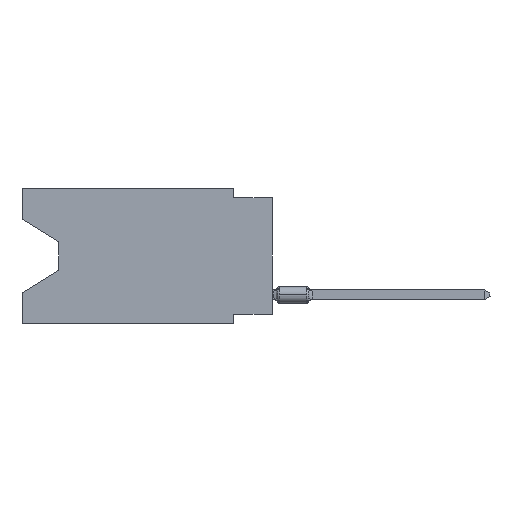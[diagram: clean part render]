
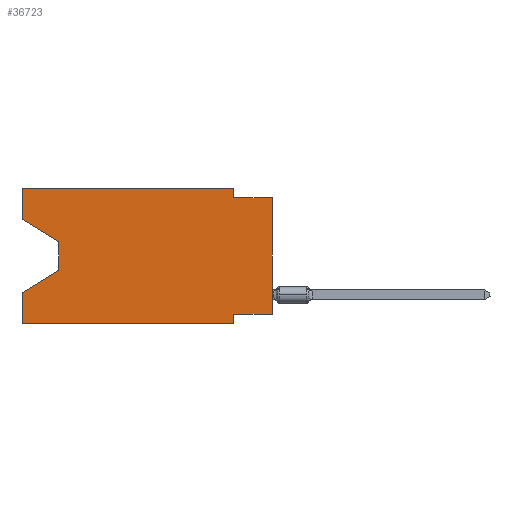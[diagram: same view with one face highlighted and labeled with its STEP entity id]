
A CAD part, left-side view. The second image highlights one B-rep face of the part: STEP entity #36723.
In plain terms, the highlighted planar face has unit normal (-1, 0, 0).
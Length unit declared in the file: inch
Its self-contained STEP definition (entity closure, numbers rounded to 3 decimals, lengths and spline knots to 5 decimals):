
#423 = EDGE_CURVE ( 'NONE', #3008, #36697, #12558, .T. ) ;
#469 = CARTESIAN_POINT ( 'NONE',  ( 0., 0.645, -0.35 ) ) ;
#643 = VECTOR ( 'NONE', #41399, 39.37008 ) ;
#1173 = CARTESIAN_POINT ( 'NONE',  ( 0., 0., -0.025 ) ) ;
#3008 = VERTEX_POINT ( 'NONE', #31290 ) ;
#3091 = CARTESIAN_POINT ( 'NONE',  ( 0., 0., -0.325 ) ) ;
#3190 = AXIS2_PLACEMENT_3D ( 'NONE', #34003, #12454, #25867 ) ;
#4300 = VECTOR ( 'NONE', #9173, 39.37008 ) ;
#5163 = CARTESIAN_POINT ( 'NONE',  ( 0., 0.1, 0. ) ) ;
#5955 = CARTESIAN_POINT ( 'NONE',  ( 0., 0.645, -0.35 ) ) ;
#6025 = ORIENTED_EDGE ( 'NONE', *, *, #23335, .T. ) ;
#6180 = VECTOR ( 'NONE', #11756, 39.37008 ) ;
#6712 = DIRECTION ( 'NONE',  ( 0., 1., 0. ) ) ;
#7247 = LINE ( 'NONE', #53947, #38737 ) ;
#7275 = LINE ( 'NONE', #50339, #6180 ) ;
#7445 = EDGE_CURVE ( 'NONE', #47457, #14428, #7247, .T. ) ;
#8168 = DIRECTION ( 'NONE',  ( 0., 0., 1. ) ) ;
#8361 = CARTESIAN_POINT ( 'NONE',  ( 0., 0.55, -0.138 ) ) ;
#8842 = LINE ( 'NONE', #29845, #42934 ) ;
#9173 = DIRECTION ( 'NONE',  ( 0., 0., 1. ) ) ;
#9623 = CARTESIAN_POINT ( 'NONE',  ( 0., 0.1, -0.025 ) ) ;
#10593 = VECTOR ( 'NONE', #22490, 39.37008 ) ;
#10892 = ORIENTED_EDGE ( 'NONE', *, *, #34061, .F. ) ;
#11405 = CARTESIAN_POINT ( 'NONE',  ( 0., 0.1, 0. ) ) ;
#11756 = DIRECTION ( 'NONE',  ( 0., 0., 1. ) ) ;
#11951 = LINE ( 'NONE', #11405, #35659 ) ;
#12297 = VECTOR ( 'NONE', #46953, 39.37008 ) ;
#12454 = DIRECTION ( 'NONE',  ( 1., 0., 0. ) ) ;
#12558 = LINE ( 'NONE', #25692, #12297 ) ;
#13240 = VERTEX_POINT ( 'NONE', #15682 ) ;
#14311 = LINE ( 'NONE', #44204, #24326 ) ;
#14428 = VERTEX_POINT ( 'NONE', #28571 ) ;
#15682 = CARTESIAN_POINT ( 'NONE',  ( 0., 0.645, -0.08025 ) ) ;
#16799 = ORIENTED_EDGE ( 'NONE', *, *, #35615, .T. ) ;
#18815 = EDGE_CURVE ( 'NONE', #50584, #54737, #8842, .T. ) ;
#18843 = DIRECTION ( 'NONE',  ( 0., -0.855, -0.519 ) ) ;
#19098 = LINE ( 'NONE', #5955, #10593 ) ;
#19164 = VECTOR ( 'NONE', #18843, 39.37008 ) ;
#19439 = CARTESIAN_POINT ( 'NONE',  ( 0., 0.1, -0.325 ) ) ;
#20526 = VERTEX_POINT ( 'NONE', #9623 ) ;
#20781 = CARTESIAN_POINT ( 'NONE',  ( 0., 0., 0. ) ) ;
#21416 = PLANE ( 'NONE',  #3190 ) ;
#22051 = CARTESIAN_POINT ( 'NONE',  ( 0., 0.645, 0. ) ) ;
#22123 = VERTEX_POINT ( 'NONE', #3091 ) ;
#22387 = EDGE_CURVE ( 'NONE', #22123, #47457, #14311, .T. ) ;
#22490 = DIRECTION ( 'NONE',  ( 0., -1., 0. ) ) ;
#23335 = EDGE_CURVE ( 'NONE', #22123, #53284, #24431, .T. ) ;
#24326 = VECTOR ( 'NONE', #6712, 39.37008 ) ;
#24431 = LINE ( 'NONE', #20781, #27405 ) ;
#25692 = CARTESIAN_POINT ( 'NONE',  ( 0., 0.645, 0. ) ) ;
#25867 = DIRECTION ( 'NONE',  ( 0., 0., -1. ) ) ;
#26146 = ORIENTED_EDGE ( 'NONE', *, *, #18815, .T. ) ;
#26285 = EDGE_CURVE ( 'NONE', #31738, #54737, #47491, .T. ) ;
#27405 = VECTOR ( 'NONE', #8168, 39.37008 ) ;
#27510 = CARTESIAN_POINT ( 'NONE',  ( 0., 0.645, -0.08025 ) ) ;
#28259 = LINE ( 'NONE', #49783, #643 ) ;
#28518 = DIRECTION ( 'NONE',  ( 0., 0., -1. ) ) ;
#28571 = CARTESIAN_POINT ( 'NONE',  ( 0., 0.1, -0.35 ) ) ;
#29615 = CARTESIAN_POINT ( 'NONE',  ( 0., 0.55, -0.212 ) ) ;
#29845 = CARTESIAN_POINT ( 'NONE',  ( 0., 0.55, -0.212 ) ) ;
#31290 = CARTESIAN_POINT ( 'NONE',  ( 0., 0.645, 0. ) ) ;
#31397 = ORIENTED_EDGE ( 'NONE', *, *, #38402, .T. ) ;
#31738 = VERTEX_POINT ( 'NONE', #469 ) ;
#34003 = CARTESIAN_POINT ( 'NONE',  ( 0., 0.645, 0. ) ) ;
#34061 = EDGE_CURVE ( 'NONE', #20526, #53284, #46473, .T. ) ;
#35113 = ORIENTED_EDGE ( 'NONE', *, *, #423, .F. ) ;
#35615 = EDGE_CURVE ( 'NONE', #31738, #14428, #19098, .T. ) ;
#35659 = VECTOR ( 'NONE', #50275, 39.37008 ) ;
#35847 = ORIENTED_EDGE ( 'NONE', *, *, #48947, .T. ) ;
#35900 = LINE ( 'NONE', #27510, #19164 ) ;
#36697 = VERTEX_POINT ( 'NONE', #5163 ) ;
#36723 = ADVANCED_FACE ( 'NONE', ( #38464 ), #21416, .F. ) ;
#37255 = CARTESIAN_POINT ( 'NONE',  ( 0., 0., -0.025 ) ) ;
#38402 = EDGE_CURVE ( 'NONE', #54139, #50584, #28259, .T. ) ;
#38464 = FACE_OUTER_BOUND ( 'NONE', #38816, .T. ) ;
#38737 = VECTOR ( 'NONE', #28518, 39.37008 ) ;
#38792 = CARTESIAN_POINT ( 'NONE',  ( 0., 0.645, -0.26975 ) ) ;
#38816 = EDGE_LOOP ( 'NONE', ( #35847, #31397, #26146, #44099, #16799, #39534, #45571, #6025, #10892, #50976, #35113, #43178 ) ) ;
#39534 = ORIENTED_EDGE ( 'NONE', *, *, #7445, .F. ) ;
#39969 = VECTOR ( 'NONE', #54314, 39.37008 ) ;
#41399 = DIRECTION ( 'NONE',  ( 0., 0., -1. ) ) ;
#42425 = EDGE_CURVE ( 'NONE', #13240, #3008, #7275, .T. ) ;
#42774 = EDGE_CURVE ( 'NONE', #36697, #20526, #11951, .T. ) ;
#42934 = VECTOR ( 'NONE', #47444, 39.37008 ) ;
#43178 = ORIENTED_EDGE ( 'NONE', *, *, #42425, .F. ) ;
#44099 = ORIENTED_EDGE ( 'NONE', *, *, #26285, .F. ) ;
#44204 = CARTESIAN_POINT ( 'NONE',  ( 0., 0., -0.325 ) ) ;
#45571 = ORIENTED_EDGE ( 'NONE', *, *, #22387, .F. ) ;
#46473 = LINE ( 'NONE', #37255, #39969 ) ;
#46953 = DIRECTION ( 'NONE',  ( 0., -1., 0. ) ) ;
#47444 = DIRECTION ( 'NONE',  ( 0., 0.855, -0.519 ) ) ;
#47457 = VERTEX_POINT ( 'NONE', #19439 ) ;
#47491 = LINE ( 'NONE', #22051, #4300 ) ;
#48947 = EDGE_CURVE ( 'NONE', #13240, #54139, #35900, .T. ) ;
#49783 = CARTESIAN_POINT ( 'NONE',  ( 0., 0.55, -0.138 ) ) ;
#50275 = DIRECTION ( 'NONE',  ( 0., 0., -1. ) ) ;
#50339 = CARTESIAN_POINT ( 'NONE',  ( 0., 0.645, 0. ) ) ;
#50584 = VERTEX_POINT ( 'NONE', #29615 ) ;
#50976 = ORIENTED_EDGE ( 'NONE', *, *, #42774, .F. ) ;
#53284 = VERTEX_POINT ( 'NONE', #1173 ) ;
#53947 = CARTESIAN_POINT ( 'NONE',  ( 0., 0.1, -0.35 ) ) ;
#54139 = VERTEX_POINT ( 'NONE', #8361 ) ;
#54314 = DIRECTION ( 'NONE',  ( 0., -1., 0. ) ) ;
#54737 = VERTEX_POINT ( 'NONE', #38792 ) ;
